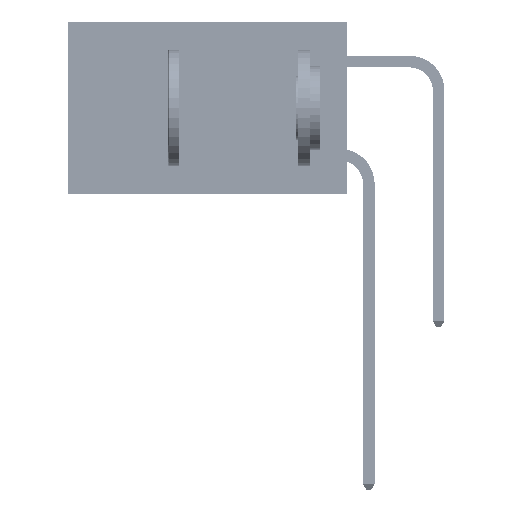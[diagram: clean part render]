
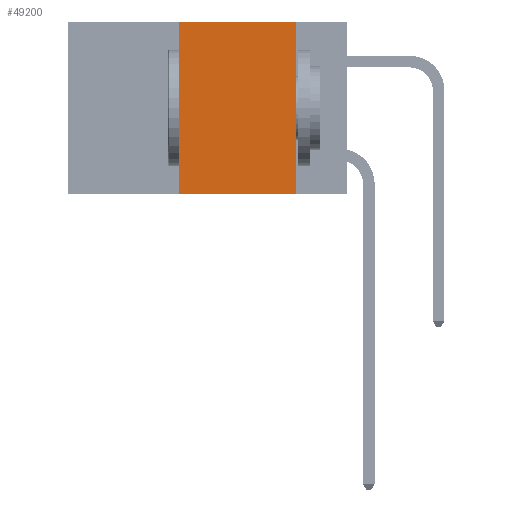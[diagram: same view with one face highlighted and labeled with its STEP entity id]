
A CAD part, left-side view. The second image highlights one B-rep face of the part: STEP entity #49200.
In plain terms, the highlighted planar face has unit normal (-1, 0, 0).
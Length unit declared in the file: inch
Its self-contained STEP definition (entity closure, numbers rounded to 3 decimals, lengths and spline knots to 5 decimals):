
#1057 = LINE ( 'NONE', #19993, #41544 ) ;
#2940 = CARTESIAN_POINT ( 'NONE',  ( 0., 0.36, 0. ) ) ;
#3097 = ORIENTED_EDGE ( 'NONE', *, *, #28056, .F. ) ;
#6184 = CARTESIAN_POINT ( 'NONE',  ( 0., 0.11, 0. ) ) ;
#6197 = VERTEX_POINT ( 'NONE', #2940 ) ;
#6381 = CARTESIAN_POINT ( 'NONE',  ( 0., 0.36, -0.37 ) ) ;
#6886 = ORIENTED_EDGE ( 'NONE', *, *, #46953, .F. ) ;
#9353 = CARTESIAN_POINT ( 'NONE',  ( 0., 0.11, 0. ) ) ;
#10226 = DIRECTION ( 'NONE',  ( 0., 0., -1. ) ) ;
#10785 = EDGE_CURVE ( 'NONE', #6197, #45164, #19703, .T. ) ;
#12792 = FACE_OUTER_BOUND ( 'NONE', #27255, .T. ) ;
#13843 = PLANE ( 'NONE',  #18398 ) ;
#14914 = CARTESIAN_POINT ( 'NONE',  ( 0., 0.6, 0. ) ) ;
#17176 = VECTOR ( 'NONE', #36970, 39.37008 ) ;
#17940 = DIRECTION ( 'NONE',  ( 1., 0., 0. ) ) ;
#18398 = AXIS2_PLACEMENT_3D ( 'NONE', #42170, #17940, #46216 ) ;
#18918 = VERTEX_POINT ( 'NONE', #6381 ) ;
#19703 = LINE ( 'NONE', #14914, #30455 ) ;
#19993 = CARTESIAN_POINT ( 'NONE',  ( 0., 0.36, 0. ) ) ;
#22935 = CARTESIAN_POINT ( 'NONE',  ( 0., 0.11, -0.37 ) ) ;
#23722 = VERTEX_POINT ( 'NONE', #22935 ) ;
#24032 = DIRECTION ( 'NONE',  ( 0., 0., 1. ) ) ;
#27255 = EDGE_LOOP ( 'NONE', ( #3097, #35406, #6886, #49903 ) ) ;
#27949 = LINE ( 'NONE', #40988, #17176 ) ;
#28056 = EDGE_CURVE ( 'NONE', #45164, #23722, #42103, .T. ) ;
#30098 = VECTOR ( 'NONE', #10226, 39.37008 ) ;
#30455 = VECTOR ( 'NONE', #43227, 39.37008 ) ;
#35406 = ORIENTED_EDGE ( 'NONE', *, *, #10785, .F. ) ;
#36970 = DIRECTION ( 'NONE',  ( 0., -1., 0. ) ) ;
#40988 = CARTESIAN_POINT ( 'NONE',  ( 0., 0.6, -0.37 ) ) ;
#41544 = VECTOR ( 'NONE', #24032, 39.37008 ) ;
#42103 = LINE ( 'NONE', #6184, #30098 ) ;
#42170 = CARTESIAN_POINT ( 'NONE',  ( 0., 0.6, 0. ) ) ;
#43227 = DIRECTION ( 'NONE',  ( 0., -1., 0. ) ) ;
#44405 = EDGE_CURVE ( 'NONE', #18918, #23722, #27949, .T. ) ;
#45164 = VERTEX_POINT ( 'NONE', #9353 ) ;
#46216 = DIRECTION ( 'NONE',  ( 0., 0., -1. ) ) ;
#46953 = EDGE_CURVE ( 'NONE', #18918, #6197, #1057, .T. ) ;
#49200 = ADVANCED_FACE ( 'NONE', ( #12792 ), #13843, .F. ) ;
#49903 = ORIENTED_EDGE ( 'NONE', *, *, #44405, .T. ) ;
